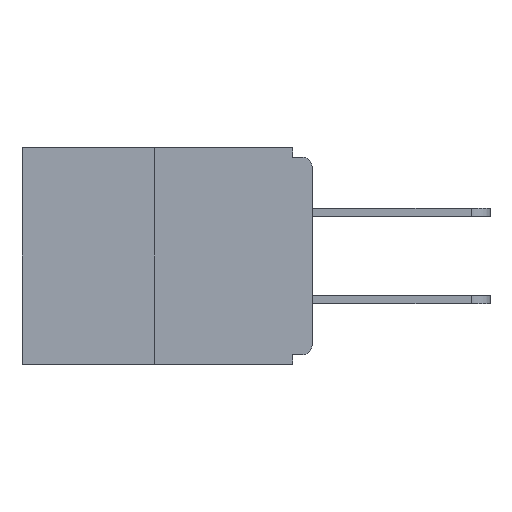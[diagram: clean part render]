
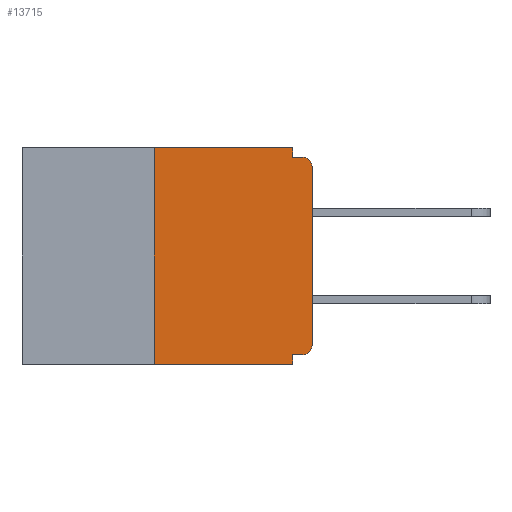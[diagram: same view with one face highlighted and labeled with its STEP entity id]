
A CAD part, left-side view. The second image highlights one B-rep face of the part: STEP entity #13715.
In plain terms, the highlighted planar face has unit normal (-1, 0, 0).
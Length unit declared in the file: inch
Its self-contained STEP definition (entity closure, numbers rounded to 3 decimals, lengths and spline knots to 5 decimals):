
#514 = DIRECTION ( 'NONE',  ( -1., 0., 0. ) ) ;
#933 = VECTOR ( 'NONE', #9046, 39.37008 ) ;
#1210 = LINE ( 'NONE', #6797, #6398 ) ;
#2008 = VERTEX_POINT ( 'NONE', #13306 ) ;
#2165 = EDGE_CURVE ( 'NONE', #7103, #6892, #1210, .T. ) ;
#2189 = CARTESIAN_POINT ( 'NONE',  ( 0., 0.46, -0.343 ) ) ;
#2288 = ORIENTED_EDGE ( 'NONE', *, *, #19914, .T. ) ;
#2316 = DIRECTION ( 'NONE',  ( 0., 1., 0. ) ) ;
#2515 = ORIENTED_EDGE ( 'NONE', *, *, #10029, .T. ) ;
#2529 = DIRECTION ( 'NONE',  ( -1., 0., 0. ) ) ;
#2544 = CARTESIAN_POINT ( 'NONE',  ( 0., 0.031, -0.015 ) ) ;
#3337 = LINE ( 'NONE', #19104, #21456 ) ;
#3769 = CARTESIAN_POINT ( 'NONE',  ( 0., 0.25, -0.343 ) ) ;
#4128 = CARTESIAN_POINT ( 'NONE',  ( 0., 0.25, 0. ) ) ;
#4159 = CARTESIAN_POINT ( 'NONE',  ( 0., 0.015, -0.015 ) ) ;
#4435 = EDGE_CURVE ( 'NONE', #2008, #4548, #11719, .T. ) ;
#4548 = VERTEX_POINT ( 'NONE', #5989 ) ;
#4644 = ORIENTED_EDGE ( 'NONE', *, *, #2165, .F. ) ;
#4701 = CIRCLE ( 'NONE', #7099, 0.015 ) ;
#4797 = VECTOR ( 'NONE', #10149, 39.37008 ) ;
#5383 = DIRECTION ( 'NONE',  ( 0., 0., 1. ) ) ;
#5945 = AXIS2_PLACEMENT_3D ( 'NONE', #17308, #10546, #21005 ) ;
#5989 = CARTESIAN_POINT ( 'NONE',  ( 0., 0.031, -0.328 ) ) ;
#6046 = CARTESIAN_POINT ( 'NONE',  ( 0., 0.015, -0.313 ) ) ;
#6099 = CARTESIAN_POINT ( 'NONE',  ( 0., 0., -0.313 ) ) ;
#6227 = VECTOR ( 'NONE', #11026, 39.37008 ) ;
#6398 = VECTOR ( 'NONE', #12054, 39.37008 ) ;
#6499 = VERTEX_POINT ( 'NONE', #4159 ) ;
#6797 = CARTESIAN_POINT ( 'NONE',  ( 0., 0.46, 0. ) ) ;
#6892 = VERTEX_POINT ( 'NONE', #12372 ) ;
#6910 = VERTEX_POINT ( 'NONE', #6099 ) ;
#7033 = EDGE_LOOP ( 'NONE', ( #4644, #21617, #14315, #8204, #17474, #13780, #2515, #2288, #22183, #9922 ) ) ;
#7099 = AXIS2_PLACEMENT_3D ( 'NONE', #21553, #514, #21706 ) ;
#7103 = VERTEX_POINT ( 'NONE', #4128 ) ;
#7161 = EDGE_CURVE ( 'NONE', #6892, #11162, #13026, .T. ) ;
#7757 = FACE_OUTER_BOUND ( 'NONE', #7033, .T. ) ;
#8204 = ORIENTED_EDGE ( 'NONE', *, *, #10981, .F. ) ;
#8573 = DIRECTION ( 'NONE',  ( 0., 0., 1. ) ) ;
#9006 = VERTEX_POINT ( 'NONE', #3769 ) ;
#9046 = DIRECTION ( 'NONE',  ( 0., -1., 0. ) ) ;
#9184 = CARTESIAN_POINT ( 'NONE',  ( 0., 0., -0.328 ) ) ;
#9642 = LINE ( 'NONE', #2189, #933 ) ;
#9922 = ORIENTED_EDGE ( 'NONE', *, *, #7161, .F. ) ;
#10029 = EDGE_CURVE ( 'NONE', #6910, #12230, #21128, .T. ) ;
#10149 = DIRECTION ( 'NONE',  ( 0., 0., -1. ) ) ;
#10426 = VECTOR ( 'NONE', #22069, 39.37008 ) ;
#10546 = DIRECTION ( 'NONE',  ( 1., 0., 0. ) ) ;
#10981 = EDGE_CURVE ( 'NONE', #4548, #18605, #12816, .T. ) ;
#11026 = DIRECTION ( 'NONE',  ( 0., 0., -1. ) ) ;
#11162 = VERTEX_POINT ( 'NONE', #2544 ) ;
#11303 = CARTESIAN_POINT ( 'NONE',  ( 0., 0., -0.015 ) ) ;
#11324 = AXIS2_PLACEMENT_3D ( 'NONE', #6046, #2529, #18316 ) ;
#11719 = LINE ( 'NONE', #9184, #18372 ) ;
#12054 = DIRECTION ( 'NONE',  ( 0., -1., 0. ) ) ;
#12230 = VERTEX_POINT ( 'NONE', #14056 ) ;
#12372 = CARTESIAN_POINT ( 'NONE',  ( 0., 0.031, 0. ) ) ;
#12816 = LINE ( 'NONE', #18255, #6227 ) ;
#13026 = LINE ( 'NONE', #19036, #4797 ) ;
#13306 = CARTESIAN_POINT ( 'NONE',  ( 0., 0.015, -0.328 ) ) ;
#13715 = ADVANCED_FACE ( 'NONE', ( #7757 ), #20928, .F. ) ;
#13780 = ORIENTED_EDGE ( 'NONE', *, *, #19357, .T. ) ;
#14012 = LINE ( 'NONE', #11303, #10426 ) ;
#14056 = CARTESIAN_POINT ( 'NONE',  ( 0., 0., -0.03 ) ) ;
#14315 = ORIENTED_EDGE ( 'NONE', *, *, #18651, .T. ) ;
#14806 = VECTOR ( 'NONE', #8573, 39.37008 ) ;
#15281 = EDGE_CURVE ( 'NONE', #9006, #7103, #3337, .T. ) ;
#17308 = CARTESIAN_POINT ( 'NONE',  ( 0., 0.46, 0. ) ) ;
#17474 = ORIENTED_EDGE ( 'NONE', *, *, #4435, .F. ) ;
#17805 = CARTESIAN_POINT ( 'NONE',  ( 0., 0.031, -0.343 ) ) ;
#18255 = CARTESIAN_POINT ( 'NONE',  ( 0., 0.031, -0.343 ) ) ;
#18316 = DIRECTION ( 'NONE',  ( 0., 0., -1. ) ) ;
#18372 = VECTOR ( 'NONE', #2316, 39.37008 ) ;
#18605 = VERTEX_POINT ( 'NONE', #17805 ) ;
#18651 = EDGE_CURVE ( 'NONE', #9006, #18605, #9642, .T. ) ;
#19036 = CARTESIAN_POINT ( 'NONE',  ( 0., 0.031, 0. ) ) ;
#19104 = CARTESIAN_POINT ( 'NONE',  ( 0., 0.25, 0. ) ) ;
#19357 = EDGE_CURVE ( 'NONE', #2008, #6910, #21726, .T. ) ;
#19459 = EDGE_CURVE ( 'NONE', #11162, #6499, #14012, .T. ) ;
#19914 = EDGE_CURVE ( 'NONE', #12230, #6499, #4701, .T. ) ;
#20853 = CARTESIAN_POINT ( 'NONE',  ( 0., 0., 0. ) ) ;
#20928 = PLANE ( 'NONE',  #5945 ) ;
#21005 = DIRECTION ( 'NONE',  ( 0., 0., -1. ) ) ;
#21128 = LINE ( 'NONE', #20853, #14806 ) ;
#21456 = VECTOR ( 'NONE', #5383, 39.37008 ) ;
#21553 = CARTESIAN_POINT ( 'NONE',  ( 0., 0.015, -0.03 ) ) ;
#21617 = ORIENTED_EDGE ( 'NONE', *, *, #15281, .F. ) ;
#21706 = DIRECTION ( 'NONE',  ( 0., 0., -1. ) ) ;
#21726 = CIRCLE ( 'NONE', #11324, 0.015 ) ;
#22069 = DIRECTION ( 'NONE',  ( 0., -1., 0. ) ) ;
#22183 = ORIENTED_EDGE ( 'NONE', *, *, #19459, .F. ) ;
